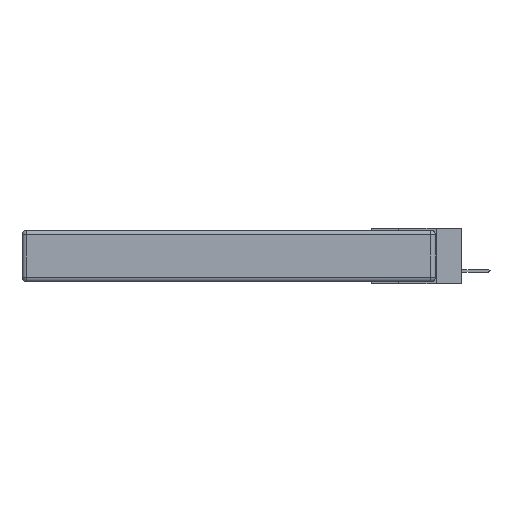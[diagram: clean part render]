
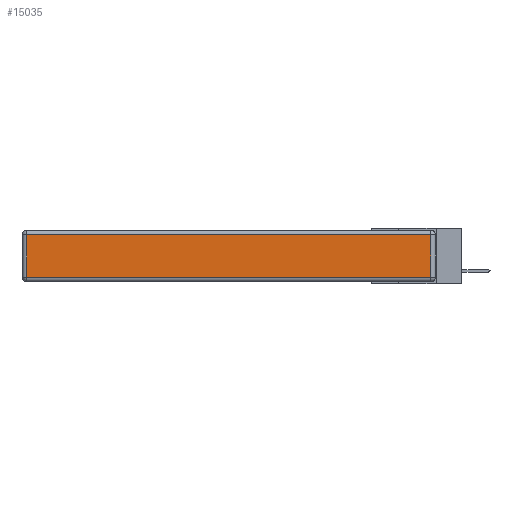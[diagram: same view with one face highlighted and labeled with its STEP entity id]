
A CAD part, left-side view. The second image highlights one B-rep face of the part: STEP entity #15035.
In plain terms, the highlighted planar face has unit normal (-1, 0, 0).
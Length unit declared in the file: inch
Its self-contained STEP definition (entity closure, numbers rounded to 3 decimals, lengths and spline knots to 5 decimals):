
#1248 = VERTEX_POINT ( 'NONE', #14160 ) ;
#1298 = CARTESIAN_POINT ( 'NONE',  ( 0., 0., -0.343 ) ) ;
#2758 = AXIS2_PLACEMENT_3D ( 'NONE', #1298, #17757, #18164 ) ;
#3527 = ORIENTED_EDGE ( 'NONE', *, *, #19590, .T. ) ;
#6157 = VECTOR ( 'NONE', #15094, 39.37008 ) ;
#8536 = CARTESIAN_POINT ( 'NONE',  ( 0., 2.72, -0.313 ) ) ;
#13751 = DIRECTION ( 'NONE',  ( 0., 0., -1. ) ) ;
#14160 = CARTESIAN_POINT ( 'NONE',  ( 0., 0.03, -0.313 ) ) ;
#15035 = ADVANCED_FACE ( 'NONE', ( #24740 ), #29634, .T. ) ;
#15094 = DIRECTION ( 'NONE',  ( 0., 0., 1. ) ) ;
#16339 = VECTOR ( 'NONE', #28496, 39.37008 ) ;
#17188 = VECTOR ( 'NONE', #22722, 39.37008 ) ;
#17757 = DIRECTION ( 'NONE',  ( -1., 0., 0. ) ) ;
#17797 = EDGE_CURVE ( 'NONE', #18402, #1248, #17909, .T. ) ;
#17839 = CARTESIAN_POINT ( 'NONE',  ( 0., 0., -0.313 ) ) ;
#17909 = LINE ( 'NONE', #17839, #17188 ) ;
#18000 = VERTEX_POINT ( 'NONE', #19062 ) ;
#18124 = LINE ( 'NONE', #20990, #27768 ) ;
#18164 = DIRECTION ( 'NONE',  ( 0., 0., 1. ) ) ;
#18402 = VERTEX_POINT ( 'NONE', #8536 ) ;
#18954 = EDGE_CURVE ( 'NONE', #18000, #25491, #30383, .T. ) ;
#19062 = CARTESIAN_POINT ( 'NONE',  ( 0., 0.03, -0.03 ) ) ;
#19590 = EDGE_CURVE ( 'NONE', #25491, #18402, #18124, .T. ) ;
#20597 = ORIENTED_EDGE ( 'NONE', *, *, #18954, .T. ) ;
#20990 = CARTESIAN_POINT ( 'NONE',  ( 0., 2.72, -0.343 ) ) ;
#22722 = DIRECTION ( 'NONE',  ( 0., -1., 0. ) ) ;
#22799 = ORIENTED_EDGE ( 'NONE', *, *, #17797, .T. ) ;
#24740 = FACE_OUTER_BOUND ( 'NONE', #29996, .T. ) ;
#25491 = VERTEX_POINT ( 'NONE', #27038 ) ;
#25650 = ORIENTED_EDGE ( 'NONE', *, *, #28802, .T. ) ;
#26253 = CARTESIAN_POINT ( 'NONE',  ( 0., 2.75, -0.03 ) ) ;
#26982 = CARTESIAN_POINT ( 'NONE',  ( 0., 0.03, -0.343 ) ) ;
#27038 = CARTESIAN_POINT ( 'NONE',  ( 0., 2.72, -0.03 ) ) ;
#27198 = LINE ( 'NONE', #26982, #6157 ) ;
#27768 = VECTOR ( 'NONE', #13751, 39.37008 ) ;
#28496 = DIRECTION ( 'NONE',  ( 0., 1., 0. ) ) ;
#28802 = EDGE_CURVE ( 'NONE', #1248, #18000, #27198, .T. ) ;
#29634 = PLANE ( 'NONE',  #2758 ) ;
#29996 = EDGE_LOOP ( 'NONE', ( #22799, #25650, #20597, #3527 ) ) ;
#30383 = LINE ( 'NONE', #26253, #16339 ) ;
